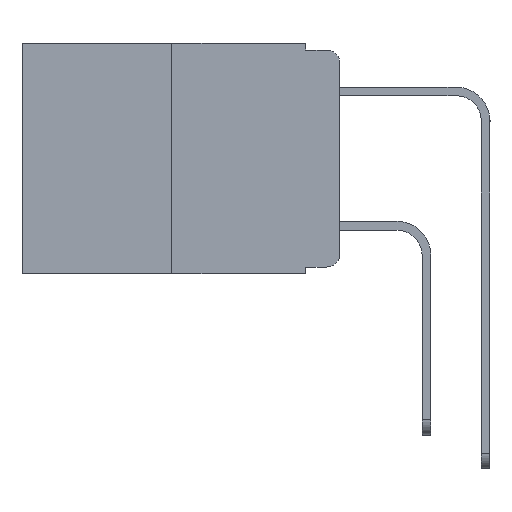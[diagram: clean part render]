
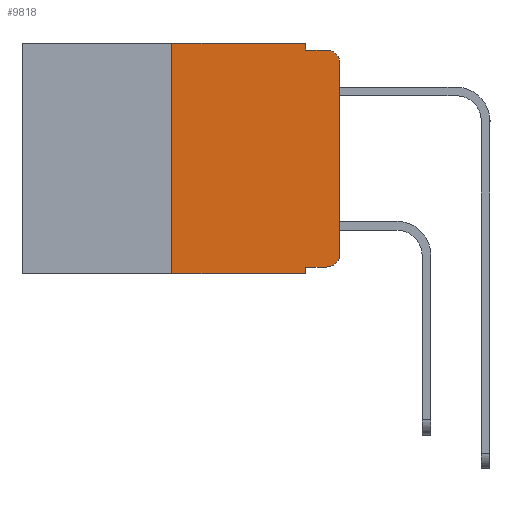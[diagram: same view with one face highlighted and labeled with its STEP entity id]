
A CAD part, left-side view. The second image highlights one B-rep face of the part: STEP entity #9818.
In plain terms, the highlighted planar face has unit normal (-1, 0, 0).
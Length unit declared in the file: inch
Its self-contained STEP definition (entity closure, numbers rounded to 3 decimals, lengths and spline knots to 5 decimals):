
#223 = DIRECTION ( 'NONE',  ( 0., -1., 0. ) ) ;
#393 = CARTESIAN_POINT ( 'NONE',  ( 0., 0.051, -0.343 ) ) ;
#483 = VERTEX_POINT ( 'NONE', #9354 ) ;
#516 = DIRECTION ( 'NONE',  ( 0., 0., -1. ) ) ;
#639 = ORIENTED_EDGE ( 'NONE', *, *, #4735, .T. ) ;
#1134 = VECTOR ( 'NONE', #5423, 39.37008 ) ;
#1244 = ORIENTED_EDGE ( 'NONE', *, *, #14203, .T. ) ;
#1321 = CARTESIAN_POINT ( 'NONE',  ( 0., 0.051, -0.01 ) ) ;
#1550 = DIRECTION ( 'NONE',  ( -1., 0., 0. ) ) ;
#1745 = CARTESIAN_POINT ( 'NONE',  ( 0., 0., 0. ) ) ;
#1835 = CARTESIAN_POINT ( 'NONE',  ( 0., 0.051, -0.333 ) ) ;
#2074 = CARTESIAN_POINT ( 'NONE',  ( 0., 0.473, 0. ) ) ;
#2262 = ORIENTED_EDGE ( 'NONE', *, *, #2341, .F. ) ;
#2341 = EDGE_CURVE ( 'NONE', #8393, #483, #11351, .T. ) ;
#2367 = VECTOR ( 'NONE', #4135, 39.37008 ) ;
#2400 = CARTESIAN_POINT ( 'NONE',  ( 0., 0., -0.313 ) ) ;
#2487 = DIRECTION ( 'NONE',  ( 0., 0., -1. ) ) ;
#2866 = CARTESIAN_POINT ( 'NONE',  ( 0., 0.051, -0.333 ) ) ;
#3006 = CARTESIAN_POINT ( 'NONE',  ( 0., 0.02, -0.313 ) ) ;
#3121 = DIRECTION ( 'NONE',  ( 0., -1., 0. ) ) ;
#3195 = VERTEX_POINT ( 'NONE', #2866 ) ;
#4135 = DIRECTION ( 'NONE',  ( 0., 0., -1. ) ) ;
#4239 = DIRECTION ( 'NONE',  ( 0., 0., -1. ) ) ;
#4505 = FACE_OUTER_BOUND ( 'NONE', #7015, .T. ) ;
#4735 = EDGE_CURVE ( 'NONE', #11310, #13562, #12787, .T. ) ;
#4812 = CIRCLE ( 'NONE', #12356, 0.02 ) ;
#4982 = DIRECTION ( 'NONE',  ( 0., 0., 1. ) ) ;
#5423 = DIRECTION ( 'NONE',  ( 0., 0., 1. ) ) ;
#5682 = VECTOR ( 'NONE', #3121, 39.37008 ) ;
#6075 = CARTESIAN_POINT ( 'NONE',  ( 0., 0.02, -0.333 ) ) ;
#6532 = EDGE_CURVE ( 'NONE', #13562, #13531, #4812, .T. ) ;
#6566 = CARTESIAN_POINT ( 'NONE',  ( 0., 0.473, 0. ) ) ;
#6579 = ORIENTED_EDGE ( 'NONE', *, *, #10815, .F. ) ;
#6709 = DIRECTION ( 'NONE',  ( 0., -1., 0. ) ) ;
#6809 = VECTOR ( 'NONE', #6709, 39.37008 ) ;
#6953 = ORIENTED_EDGE ( 'NONE', *, *, #14281, .T. ) ;
#7015 = EDGE_LOOP ( 'NONE', ( #639, #10204, #7778, #13364, #2262, #14026, #14348, #6579, #6953, #1244 ) ) ;
#7089 = VERTEX_POINT ( 'NONE', #6075 ) ;
#7116 = EDGE_CURVE ( 'NONE', #483, #13708, #12730, .T. ) ;
#7461 = CARTESIAN_POINT ( 'NONE',  ( 0., 0.051, -0.01 ) ) ;
#7714 = DIRECTION ( 'NONE',  ( 1., 0., 0. ) ) ;
#7778 = ORIENTED_EDGE ( 'NONE', *, *, #10697, .F. ) ;
#7922 = CARTESIAN_POINT ( 'NONE',  ( 0., 0., -0.03 ) ) ;
#7934 = CARTESIAN_POINT ( 'NONE',  ( 0., 0.25, 0. ) ) ;
#8128 = VERTEX_POINT ( 'NONE', #393 ) ;
#8393 = VERTEX_POINT ( 'NONE', #7934 ) ;
#8396 = CARTESIAN_POINT ( 'NONE',  ( 0., 0.25, -0.343 ) ) ;
#8543 = CARTESIAN_POINT ( 'NONE',  ( 0., 0.02, -0.03 ) ) ;
#8892 = CIRCLE ( 'NONE', #9357, 0.02 ) ;
#9240 = LINE ( 'NONE', #13039, #6809 ) ;
#9354 = CARTESIAN_POINT ( 'NONE',  ( 0., 0.051, 0. ) ) ;
#9357 = AXIS2_PLACEMENT_3D ( 'NONE', #3006, #10797, #4239 ) ;
#9555 = VERTEX_POINT ( 'NONE', #8396 ) ;
#9564 = DIRECTION ( 'NONE',  ( 0., 0., -1. ) ) ;
#9818 = ADVANCED_FACE ( 'NONE', ( #4505 ), #11870, .F. ) ;
#9903 = VECTOR ( 'NONE', #2487, 39.37008 ) ;
#10005 = DIRECTION ( 'NONE',  ( 0., -1., 0. ) ) ;
#10204 = ORIENTED_EDGE ( 'NONE', *, *, #6532, .T. ) ;
#10230 = VECTOR ( 'NONE', #4982, 39.37008 ) ;
#10697 = EDGE_CURVE ( 'NONE', #13708, #13531, #12283, .T. ) ;
#10705 = CARTESIAN_POINT ( 'NONE',  ( 0., 0.051, 0. ) ) ;
#10797 = DIRECTION ( 'NONE',  ( -1., 0., 0. ) ) ;
#10815 = EDGE_CURVE ( 'NONE', #3195, #8128, #11284, .T. ) ;
#11284 = LINE ( 'NONE', #10705, #2367 ) ;
#11310 = VERTEX_POINT ( 'NONE', #2400 ) ;
#11351 = LINE ( 'NONE', #2074, #12018 ) ;
#11354 = LINE ( 'NONE', #1835, #5682 ) ;
#11870 = PLANE ( 'NONE',  #12195 ) ;
#12018 = VECTOR ( 'NONE', #10005, 39.37008 ) ;
#12195 = AXIS2_PLACEMENT_3D ( 'NONE', #6566, #7714, #516 ) ;
#12283 = LINE ( 'NONE', #7461, #12626 ) ;
#12356 = AXIS2_PLACEMENT_3D ( 'NONE', #8543, #1550, #9564 ) ;
#12440 = CARTESIAN_POINT ( 'NONE',  ( 0., 0.051, 0. ) ) ;
#12596 = EDGE_CURVE ( 'NONE', #9555, #8128, #9240, .T. ) ;
#12626 = VECTOR ( 'NONE', #223, 39.37008 ) ;
#12730 = LINE ( 'NONE', #12440, #9903 ) ;
#12787 = LINE ( 'NONE', #1745, #1134 ) ;
#13034 = EDGE_CURVE ( 'NONE', #9555, #8393, #13073, .T. ) ;
#13039 = CARTESIAN_POINT ( 'NONE',  ( 0., 0.473, -0.343 ) ) ;
#13073 = LINE ( 'NONE', #13532, #10230 ) ;
#13161 = CARTESIAN_POINT ( 'NONE',  ( 0., 0.02, -0.01 ) ) ;
#13364 = ORIENTED_EDGE ( 'NONE', *, *, #7116, .F. ) ;
#13531 = VERTEX_POINT ( 'NONE', #13161 ) ;
#13532 = CARTESIAN_POINT ( 'NONE',  ( 0., 0.25, 0. ) ) ;
#13562 = VERTEX_POINT ( 'NONE', #7922 ) ;
#13708 = VERTEX_POINT ( 'NONE', #1321 ) ;
#14026 = ORIENTED_EDGE ( 'NONE', *, *, #13034, .F. ) ;
#14203 = EDGE_CURVE ( 'NONE', #7089, #11310, #8892, .T. ) ;
#14281 = EDGE_CURVE ( 'NONE', #3195, #7089, #11354, .T. ) ;
#14348 = ORIENTED_EDGE ( 'NONE', *, *, #12596, .T. ) ;
